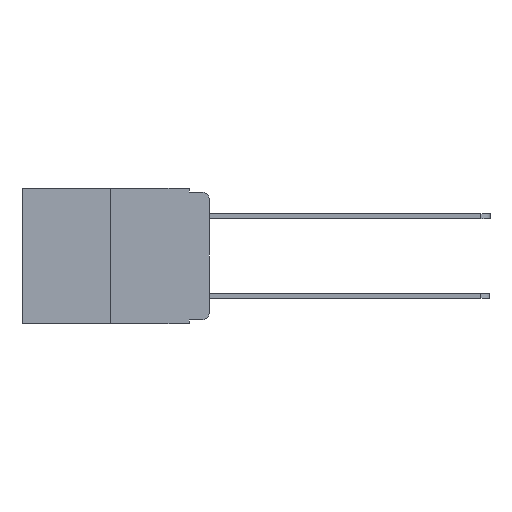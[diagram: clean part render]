
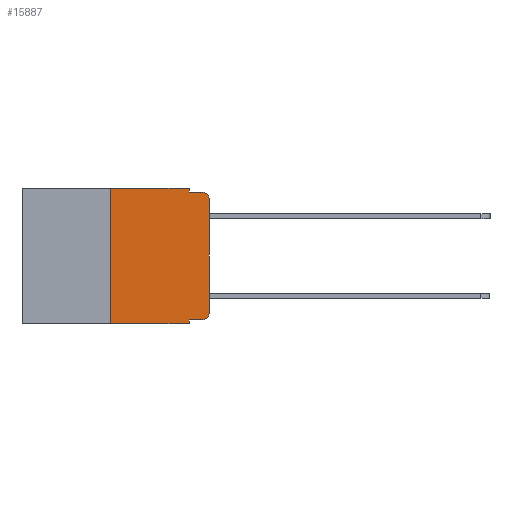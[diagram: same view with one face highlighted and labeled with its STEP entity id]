
A CAD part, left-side view. The second image highlights one B-rep face of the part: STEP entity #15887.
In plain terms, the highlighted planar face has unit normal (-1, 0, 0).
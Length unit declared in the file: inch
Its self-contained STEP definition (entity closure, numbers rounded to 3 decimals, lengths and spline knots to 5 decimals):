
#494 = VECTOR ( 'NONE', #8027, 39.37008 ) ;
#924 = DIRECTION ( 'NONE',  ( -1., 0., 0. ) ) ;
#1076 = CARTESIAN_POINT ( 'NONE',  ( 0., 0.051, -0.01 ) ) ;
#1085 = DIRECTION ( 'NONE',  ( 0., 0., -1. ) ) ;
#1308 = AXIS2_PLACEMENT_3D ( 'NONE', #11280, #924, #12945 ) ;
#1449 = LINE ( 'NONE', #16243, #6117 ) ;
#1533 = VERTEX_POINT ( 'NONE', #8324 ) ;
#1630 = LINE ( 'NONE', #16061, #11372 ) ;
#1700 = PLANE ( 'NONE',  #14822 ) ;
#1798 = CARTESIAN_POINT ( 'NONE',  ( 0., 0.25, 0. ) ) ;
#2001 = LINE ( 'NONE', #1076, #6133 ) ;
#2063 = CARTESIAN_POINT ( 'NONE',  ( 0., 0.051, 0. ) ) ;
#2408 = DIRECTION ( 'NONE',  ( 0., -1., 0. ) ) ;
#2792 = DIRECTION ( 'NONE',  ( 0., -1., 0. ) ) ;
#2924 = VECTOR ( 'NONE', #20379, 39.37008 ) ;
#3338 = AXIS2_PLACEMENT_3D ( 'NONE', #4810, #16533, #6565 ) ;
#3482 = ORIENTED_EDGE ( 'NONE', *, *, #8058, .T. ) ;
#3923 = VECTOR ( 'NONE', #19042, 39.37008 ) ;
#4007 = ORIENTED_EDGE ( 'NONE', *, *, #13283, .F. ) ;
#4701 = EDGE_CURVE ( 'NONE', #19731, #8806, #5686, .T. ) ;
#4810 = CARTESIAN_POINT ( 'NONE',  ( 0., 0.02, -0.313 ) ) ;
#5050 = CARTESIAN_POINT ( 'NONE',  ( 0., 0.051, -0.333 ) ) ;
#5149 = VERTEX_POINT ( 'NONE', #6350 ) ;
#5238 = DIRECTION ( 'NONE',  ( 1., 0., 0. ) ) ;
#5645 = EDGE_CURVE ( 'NONE', #19731, #17066, #10733, .T. ) ;
#5686 = LINE ( 'NONE', #1798, #494 ) ;
#6117 = VECTOR ( 'NONE', #1085, 39.37008 ) ;
#6133 = VECTOR ( 'NONE', #2792, 39.37008 ) ;
#6185 = VECTOR ( 'NONE', #2408, 39.37008 ) ;
#6350 = CARTESIAN_POINT ( 'NONE',  ( 0., 0.051, -0.333 ) ) ;
#6565 = DIRECTION ( 'NONE',  ( 0., 0., -1. ) ) ;
#6784 = DIRECTION ( 'NONE',  ( 0., -1., 0. ) ) ;
#7163 = ORIENTED_EDGE ( 'NONE', *, *, #11638, .F. ) ;
#7356 = EDGE_CURVE ( 'NONE', #19752, #14044, #1630, .T. ) ;
#7939 = CARTESIAN_POINT ( 'NONE',  ( 0., 0., -0.03 ) ) ;
#8027 = DIRECTION ( 'NONE',  ( 0., 0., 1. ) ) ;
#8058 = EDGE_CURVE ( 'NONE', #14044, #1533, #18161, .T. ) ;
#8324 = CARTESIAN_POINT ( 'NONE',  ( 0., 0.02, -0.01 ) ) ;
#8689 = FACE_OUTER_BOUND ( 'NONE', #19272, .T. ) ;
#8806 = VERTEX_POINT ( 'NONE', #13050 ) ;
#9172 = EDGE_CURVE ( 'NONE', #5149, #17066, #15408, .T. ) ;
#10337 = CARTESIAN_POINT ( 'NONE',  ( 0., 0.051, 0. ) ) ;
#10431 = CARTESIAN_POINT ( 'NONE',  ( 0., 0.051, -0.343 ) ) ;
#10705 = VERTEX_POINT ( 'NONE', #10337 ) ;
#10733 = LINE ( 'NONE', #11621, #6185 ) ;
#10976 = CARTESIAN_POINT ( 'NONE',  ( 0., 0.473, 0. ) ) ;
#11280 = CARTESIAN_POINT ( 'NONE',  ( 0., 0.02, -0.03 ) ) ;
#11372 = VECTOR ( 'NONE', #17669, 39.37008 ) ;
#11621 = CARTESIAN_POINT ( 'NONE',  ( 0., 0.473, -0.343 ) ) ;
#11638 = EDGE_CURVE ( 'NONE', #19213, #1533, #2001, .T. ) ;
#11972 = LINE ( 'NONE', #5050, #19520 ) ;
#12049 = CARTESIAN_POINT ( 'NONE',  ( 0., 0.25, -0.343 ) ) ;
#12258 = ORIENTED_EDGE ( 'NONE', *, *, #18215, .T. ) ;
#12294 = CARTESIAN_POINT ( 'NONE',  ( 0., 0.051, -0.01 ) ) ;
#12945 = DIRECTION ( 'NONE',  ( 0., 0., -1. ) ) ;
#13050 = CARTESIAN_POINT ( 'NONE',  ( 0., 0.25, 0. ) ) ;
#13283 = EDGE_CURVE ( 'NONE', #8806, #10705, #13513, .T. ) ;
#13513 = LINE ( 'NONE', #10976, #3923 ) ;
#13684 = CARTESIAN_POINT ( 'NONE',  ( 0., 0.473, 0. ) ) ;
#14044 = VERTEX_POINT ( 'NONE', #7939 ) ;
#14801 = ORIENTED_EDGE ( 'NONE', *, *, #9172, .F. ) ;
#14822 = AXIS2_PLACEMENT_3D ( 'NONE', #13684, #5238, #16908 ) ;
#15408 = LINE ( 'NONE', #2063, #2924 ) ;
#15887 = ADVANCED_FACE ( 'NONE', ( #8689 ), #1700, .F. ) ;
#16061 = CARTESIAN_POINT ( 'NONE',  ( 0., 0., 0. ) ) ;
#16139 = ORIENTED_EDGE ( 'NONE', *, *, #7356, .T. ) ;
#16243 = CARTESIAN_POINT ( 'NONE',  ( 0., 0.051, 0. ) ) ;
#16421 = ORIENTED_EDGE ( 'NONE', *, *, #18968, .T. ) ;
#16533 = DIRECTION ( 'NONE',  ( -1., 0., 0. ) ) ;
#16561 = CARTESIAN_POINT ( 'NONE',  ( 0., 0.02, -0.333 ) ) ;
#16908 = DIRECTION ( 'NONE',  ( 0., 0., -1. ) ) ;
#17066 = VERTEX_POINT ( 'NONE', #10431 ) ;
#17090 = ORIENTED_EDGE ( 'NONE', *, *, #5645, .T. ) ;
#17532 = VERTEX_POINT ( 'NONE', #16561 ) ;
#17669 = DIRECTION ( 'NONE',  ( 0., 0., 1. ) ) ;
#17716 = ORIENTED_EDGE ( 'NONE', *, *, #18033, .F. ) ;
#17730 = CIRCLE ( 'NONE', #3338, 0.02 ) ;
#18033 = EDGE_CURVE ( 'NONE', #10705, #19213, #1449, .T. ) ;
#18161 = CIRCLE ( 'NONE', #1308, 0.02 ) ;
#18215 = EDGE_CURVE ( 'NONE', #5149, #17532, #11972, .T. ) ;
#18337 = ORIENTED_EDGE ( 'NONE', *, *, #4701, .F. ) ;
#18532 = CARTESIAN_POINT ( 'NONE',  ( 0., 0., -0.313 ) ) ;
#18968 = EDGE_CURVE ( 'NONE', #17532, #19752, #17730, .T. ) ;
#19042 = DIRECTION ( 'NONE',  ( 0., -1., 0. ) ) ;
#19213 = VERTEX_POINT ( 'NONE', #12294 ) ;
#19272 = EDGE_LOOP ( 'NONE', ( #16139, #3482, #7163, #17716, #4007, #18337, #17090, #14801, #12258, #16421 ) ) ;
#19520 = VECTOR ( 'NONE', #6784, 39.37008 ) ;
#19731 = VERTEX_POINT ( 'NONE', #12049 ) ;
#19752 = VERTEX_POINT ( 'NONE', #18532 ) ;
#20379 = DIRECTION ( 'NONE',  ( 0., 0., -1. ) ) ;
